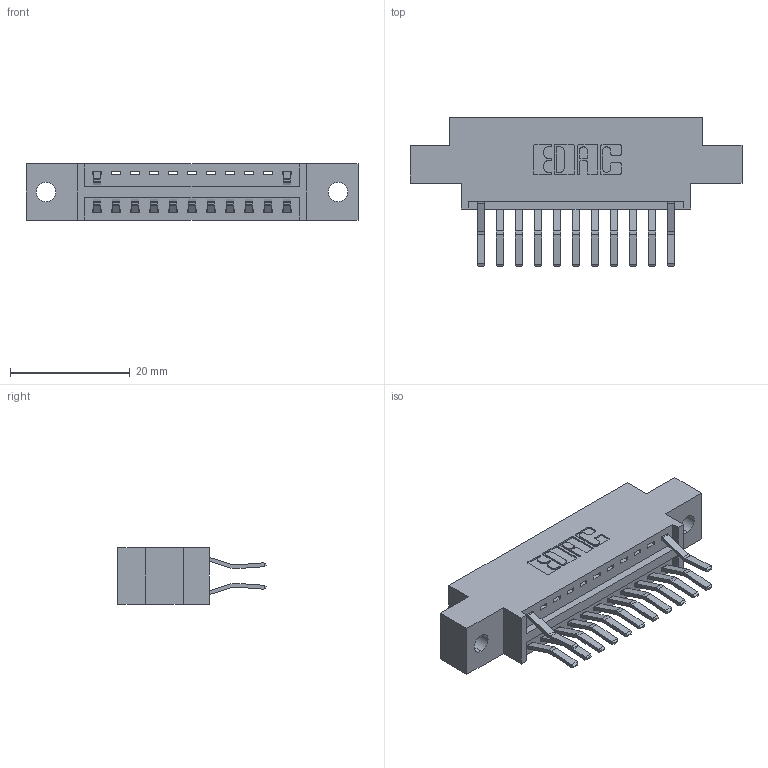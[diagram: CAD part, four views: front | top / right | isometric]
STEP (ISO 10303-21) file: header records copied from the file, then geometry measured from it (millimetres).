
FILE_DESCRIPTION (( 'STEP AP203' ), '1' );
FILE_NAME ('346-022-560-802.STEP', '2018-08-21T01:29:50', ( '' ), ( '' ), 'SwSTEP 2.0', 'SolidWorks 2016', '' );
FILE_SCHEMA (( 'CONFIG_CONTROL_DESIGN' ));
Length unit declared in the file: inch
Products named in the file (3): 345-292-001_560 Tail; 346-022-560-802; 346 Part_0.170 Offset - 0.128 Dia
Assembly tree (14 placements, depth 2):
  346-022-560-802
    346 Part_0.170 Offset - 0.128 Dia
    345-292-001_560 Tail  x13
Bounding box: 55.5 x 24.78 x 9.4 mm (x, y, z)
Volume: 4984 mm3; surface area: 6034.2 mm2
Topology: 14 solids, 14 shells, 882 faces, 2623 edges, 1730 vertices
Faces by surface type: plane 580, cylinder 302
Entity records: 11287 total; most frequent: CARTESIAN_POINT 1943, ORIENTED_EDGE 1886, DIRECTION 1757, EDGE_CURVE 943, VECTOR 763, LINE 763, VERTEX_POINT 626, AXIS2_PLACEMENT_3D 497
